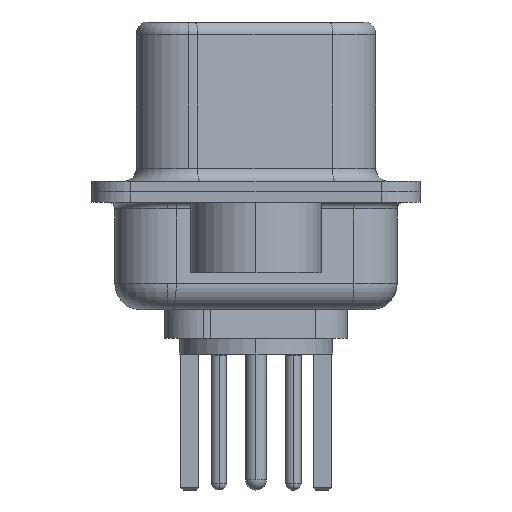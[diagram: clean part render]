
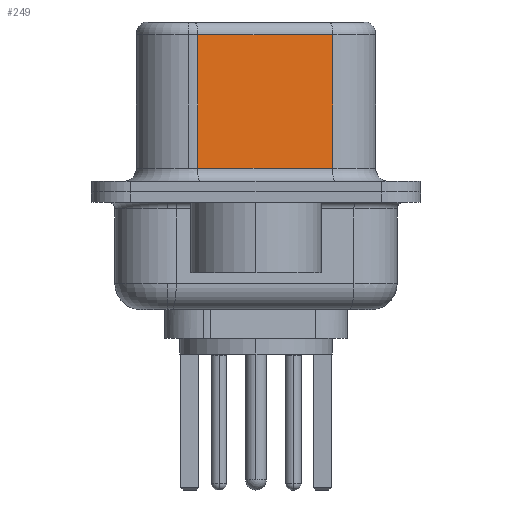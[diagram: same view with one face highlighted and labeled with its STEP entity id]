
A CAD part, left-side view. The second image highlights one B-rep face of the part: STEP entity #249.
In plain terms, the highlighted planar face has unit normal (-0.985, -0.174, 0).
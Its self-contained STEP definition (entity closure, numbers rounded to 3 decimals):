
#249 = ADVANCED_FACE ( 'NONE', ( #15613 ), #1290, .F. ) ;
#275 = VECTOR ( 'NONE', #13654, 1000. ) ;
#912 = CARTESIAN_POINT ( 'NONE',  ( 4.585, -2.927, 6.52 ) ) ;
#1064 = VERTEX_POINT ( 'NONE', #11728 ) ;
#1091 = CARTESIAN_POINT ( 'NONE',  ( 4.585, -2.927, 0.9 ) ) ;
#1290 = PLANE ( 'NONE',  #6963 ) ;
#1352 = EDGE_CURVE ( 'NONE', #1064, #18515, #18450, .T. ) ;
#2487 = CARTESIAN_POINT ( 'NONE',  ( 4.585, -2.927, 0.9 ) ) ;
#3216 = CARTESIAN_POINT ( 'NONE',  ( 3.675, 2.233, 6.52 ) ) ;
#5285 = DIRECTION ( 'NONE',  ( 0.174, -0.985, 0. ) ) ;
#5419 = ORIENTED_EDGE ( 'NONE', *, *, #15313, .T. ) ;
#6666 = CARTESIAN_POINT ( 'NONE',  ( 4.585, -2.927, 6.52 ) ) ;
#6751 = DIRECTION ( 'NONE',  ( -0.174, 0.985, 0. ) ) ;
#6879 = ORIENTED_EDGE ( 'NONE', *, *, #15773, .T. ) ;
#6910 = DIRECTION ( 'NONE',  ( 0.985, 0.174, 0. ) ) ;
#6963 = AXIS2_PLACEMENT_3D ( 'NONE', #6666, #6910, #16045 ) ;
#6991 = LINE ( 'NONE', #3216, #21026 ) ;
#8428 = VERTEX_POINT ( 'NONE', #14369 ) ;
#8709 = EDGE_LOOP ( 'NONE', ( #14430, #6879, #5419, #17372 ) ) ;
#9260 = VECTOR ( 'NONE', #6751, 1000. ) ;
#9830 = LINE ( 'NONE', #19533, #9260 ) ;
#9942 = LINE ( 'NONE', #912, #275 ) ;
#11728 = CARTESIAN_POINT ( 'NONE',  ( 3.675, 2.233, 0.9 ) ) ;
#11997 = EDGE_CURVE ( 'NONE', #8428, #18515, #9942, .T. ) ;
#12303 = DIRECTION ( 'NONE',  ( 0., 0., -1. ) ) ;
#13024 = VECTOR ( 'NONE', #5285, 1000. ) ;
#13654 = DIRECTION ( 'NONE',  ( 0., 0., -1. ) ) ;
#14369 = CARTESIAN_POINT ( 'NONE',  ( 4.585, -2.927, 6.02 ) ) ;
#14430 = ORIENTED_EDGE ( 'NONE', *, *, #11997, .F. ) ;
#15313 = EDGE_CURVE ( 'NONE', #15835, #1064, #6991, .T. ) ;
#15613 = FACE_OUTER_BOUND ( 'NONE', #8709, .T. ) ;
#15773 = EDGE_CURVE ( 'NONE', #8428, #15835, #9830, .T. ) ;
#15835 = VERTEX_POINT ( 'NONE', #21542 ) ;
#16045 = DIRECTION ( 'NONE',  ( -0.174, 0.985, 0. ) ) ;
#17372 = ORIENTED_EDGE ( 'NONE', *, *, #1352, .T. ) ;
#18450 = LINE ( 'NONE', #1091, #13024 ) ;
#18515 = VERTEX_POINT ( 'NONE', #2487 ) ;
#19533 = CARTESIAN_POINT ( 'NONE',  ( 4.585, -2.927, 6.02 ) ) ;
#21026 = VECTOR ( 'NONE', #12303, 1000. ) ;
#21542 = CARTESIAN_POINT ( 'NONE',  ( 3.675, 2.233, 6.02 ) ) ;
